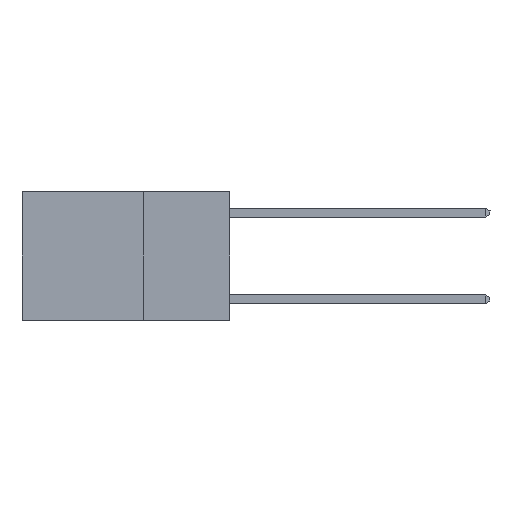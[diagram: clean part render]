
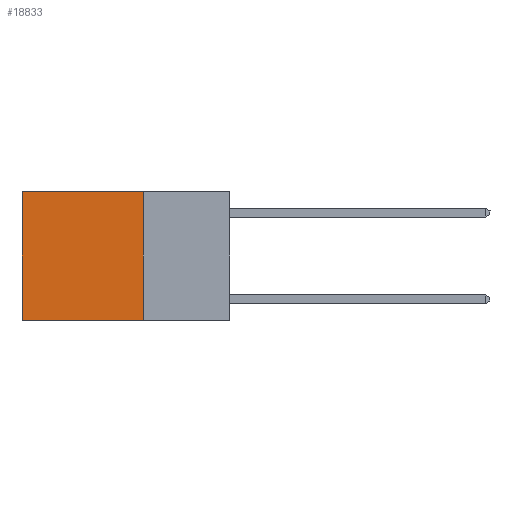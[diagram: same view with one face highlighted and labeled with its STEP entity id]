
A CAD part, left-side view. The second image highlights one B-rep face of the part: STEP entity #18833.
In plain terms, the highlighted planar face has unit normal (-1, 0, 0).
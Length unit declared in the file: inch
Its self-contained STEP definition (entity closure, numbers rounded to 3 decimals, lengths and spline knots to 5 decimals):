
#228 = VERTEX_POINT ( 'NONE', #956 ) ;
#407 = EDGE_CURVE ( 'NONE', #2749, #8652, #10068, .T. ) ;
#956 = CARTESIAN_POINT ( 'NONE',  ( 0.2625, 0.25, -0.37 ) ) ;
#2749 = VERTEX_POINT ( 'NONE', #10874 ) ;
#2902 = CARTESIAN_POINT ( 'NONE',  ( 0.2625, 0.25, 0. ) ) ;
#2968 = CARTESIAN_POINT ( 'NONE',  ( 0.2625, 0.25, 0. ) ) ;
#4428 = DIRECTION ( 'NONE',  ( 0., 0., -1. ) ) ;
#4606 = VERTEX_POINT ( 'NONE', #20069 ) ;
#4791 = CARTESIAN_POINT ( 'NONE',  ( 0.2625, 0.6, 0. ) ) ;
#5384 = VECTOR ( 'NONE', #11310, 39.37008 ) ;
#6571 = DIRECTION ( 'NONE',  ( 0., 1., 0. ) ) ;
#7236 = ORIENTED_EDGE ( 'NONE', *, *, #20714, .F. ) ;
#7812 = LINE ( 'NONE', #21927, #19128 ) ;
#7933 = CARTESIAN_POINT ( 'NONE',  ( 0.2625, 0.6, 0. ) ) ;
#8652 = VERTEX_POINT ( 'NONE', #4791 ) ;
#9022 = EDGE_CURVE ( 'NONE', #228, #4606, #7812, .T. ) ;
#9941 = PLANE ( 'NONE',  #21054 ) ;
#10065 = ORIENTED_EDGE ( 'NONE', *, *, #9022, .F. ) ;
#10068 = LINE ( 'NONE', #22043, #21105 ) ;
#10533 = ORIENTED_EDGE ( 'NONE', *, *, #14230, .T. ) ;
#10874 = CARTESIAN_POINT ( 'NONE',  ( 0.2625, 0.25, 0. ) ) ;
#11029 = ORIENTED_EDGE ( 'NONE', *, *, #407, .T. ) ;
#11310 = DIRECTION ( 'NONE',  ( 0., 0., -1. ) ) ;
#11528 = LINE ( 'NONE', #7933, #5384 ) ;
#14230 = EDGE_CURVE ( 'NONE', #8652, #4606, #11528, .T. ) ;
#14951 = DIRECTION ( 'NONE',  ( 0., 0., -1. ) ) ;
#15437 = EDGE_LOOP ( 'NONE', ( #10533, #10065, #7236, #11029 ) ) ;
#16591 = DIRECTION ( 'NONE',  ( 1., 0., 0. ) ) ;
#17903 = LINE ( 'NONE', #2902, #18586 ) ;
#18311 = DIRECTION ( 'NONE',  ( 0., 1., 0. ) ) ;
#18586 = VECTOR ( 'NONE', #14951, 39.37008 ) ;
#18833 = ADVANCED_FACE ( 'NONE', ( #20095 ), #9941, .F. ) ;
#19128 = VECTOR ( 'NONE', #18311, 39.37008 ) ;
#20069 = CARTESIAN_POINT ( 'NONE',  ( 0.2625, 0.6, -0.37 ) ) ;
#20095 = FACE_OUTER_BOUND ( 'NONE', #15437, .T. ) ;
#20714 = EDGE_CURVE ( 'NONE', #2749, #228, #17903, .T. ) ;
#21054 = AXIS2_PLACEMENT_3D ( 'NONE', #2968, #16591, #4428 ) ;
#21105 = VECTOR ( 'NONE', #6571, 39.37008 ) ;
#21927 = CARTESIAN_POINT ( 'NONE',  ( 0.2625, 0.25, -0.37 ) ) ;
#22043 = CARTESIAN_POINT ( 'NONE',  ( 0.2625, 0.25, 0. ) ) ;
